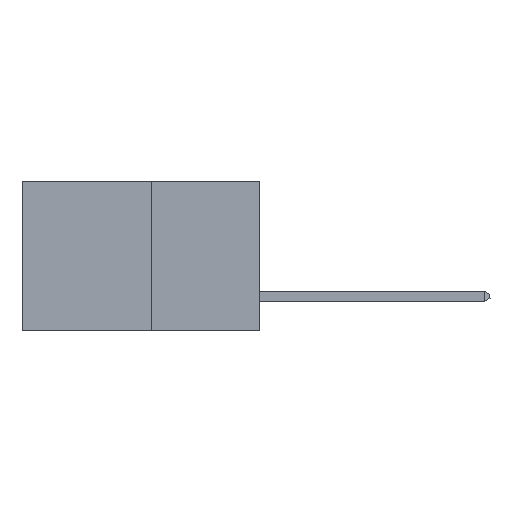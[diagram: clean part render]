
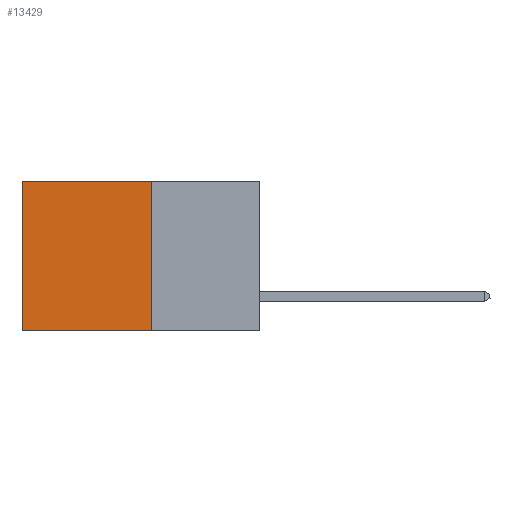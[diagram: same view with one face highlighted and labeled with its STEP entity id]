
A CAD part, left-side view. The second image highlights one B-rep face of the part: STEP entity #13429.
In plain terms, the highlighted planar face has unit normal (-1, 0, 0).
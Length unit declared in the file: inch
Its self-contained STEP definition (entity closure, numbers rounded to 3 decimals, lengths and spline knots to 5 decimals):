
#276 = FACE_OUTER_BOUND ( 'NONE', #3461, .T. ) ;
#540 = ORIENTED_EDGE ( 'NONE', *, *, #7315, .F. ) ;
#578 = CARTESIAN_POINT ( 'NONE',  ( 0.277, 0.27, 0. ) ) ;
#1558 = VECTOR ( 'NONE', #10661, 39.37008 ) ;
#2522 = ORIENTED_EDGE ( 'NONE', *, *, #7175, .T. ) ;
#2806 = DIRECTION ( 'NONE',  ( 0., 1., 0. ) ) ;
#3461 = EDGE_LOOP ( 'NONE', ( #2522, #7483, #540, #7130 ) ) ;
#3650 = VECTOR ( 'NONE', #8414, 39.37008 ) ;
#4817 = LINE ( 'NONE', #8628, #1558 ) ;
#5284 = DIRECTION ( 'NONE',  ( 0., 0., -1. ) ) ;
#6083 = AXIS2_PLACEMENT_3D ( 'NONE', #6331, #11524, #5284 ) ;
#6306 = EDGE_CURVE ( 'NONE', #8834, #12700, #6911, .T. ) ;
#6331 = CARTESIAN_POINT ( 'NONE',  ( 0.277, 0.27, -0.37 ) ) ;
#6349 = CARTESIAN_POINT ( 'NONE',  ( 0.277, 0.59, -0.37 ) ) ;
#6911 = LINE ( 'NONE', #12023, #9330 ) ;
#7067 = VERTEX_POINT ( 'NONE', #10329 ) ;
#7130 = ORIENTED_EDGE ( 'NONE', *, *, #7677, .T. ) ;
#7175 = EDGE_CURVE ( 'NONE', #7819, #12700, #9307, .T. ) ;
#7315 = EDGE_CURVE ( 'NONE', #7067, #8834, #4817, .T. ) ;
#7483 = ORIENTED_EDGE ( 'NONE', *, *, #6306, .F. ) ;
#7677 = EDGE_CURVE ( 'NONE', #7067, #7819, #13462, .T. ) ;
#7819 = VERTEX_POINT ( 'NONE', #8399 ) ;
#8002 = VECTOR ( 'NONE', #2806, 39.37008 ) ;
#8399 = CARTESIAN_POINT ( 'NONE',  ( 0.277, 0.59, 0. ) ) ;
#8414 = DIRECTION ( 'NONE',  ( 0., 0., -1. ) ) ;
#8628 = CARTESIAN_POINT ( 'NONE',  ( 0.277, 0.27, -0.37 ) ) ;
#8834 = VERTEX_POINT ( 'NONE', #10031 ) ;
#9307 = LINE ( 'NONE', #6349, #3650 ) ;
#9330 = VECTOR ( 'NONE', #13049, 39.37008 ) ;
#10031 = CARTESIAN_POINT ( 'NONE',  ( 0.277, 0.27, -0.37 ) ) ;
#10327 = CARTESIAN_POINT ( 'NONE',  ( 0.277, 0.59, -0.37 ) ) ;
#10329 = CARTESIAN_POINT ( 'NONE',  ( 0.277, 0.27, 0. ) ) ;
#10493 = PLANE ( 'NONE',  #6083 ) ;
#10661 = DIRECTION ( 'NONE',  ( 0., 0., -1. ) ) ;
#11524 = DIRECTION ( 'NONE',  ( 1., 0., 0. ) ) ;
#12023 = CARTESIAN_POINT ( 'NONE',  ( 0.277, 0.27, -0.37 ) ) ;
#12700 = VERTEX_POINT ( 'NONE', #10327 ) ;
#13049 = DIRECTION ( 'NONE',  ( 0., 1., 0. ) ) ;
#13429 = ADVANCED_FACE ( 'NONE', ( #276 ), #10493, .F. ) ;
#13462 = LINE ( 'NONE', #578, #8002 ) ;
